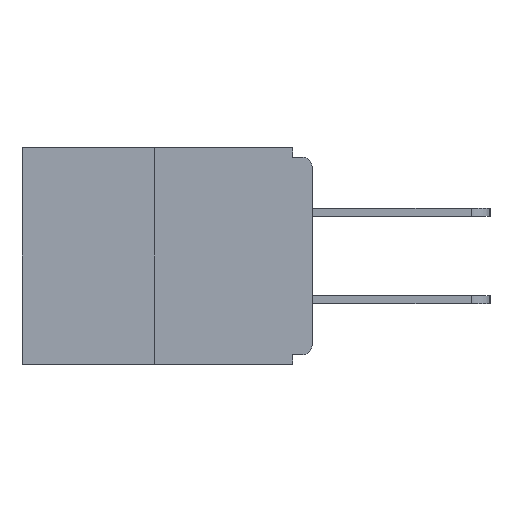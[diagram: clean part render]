
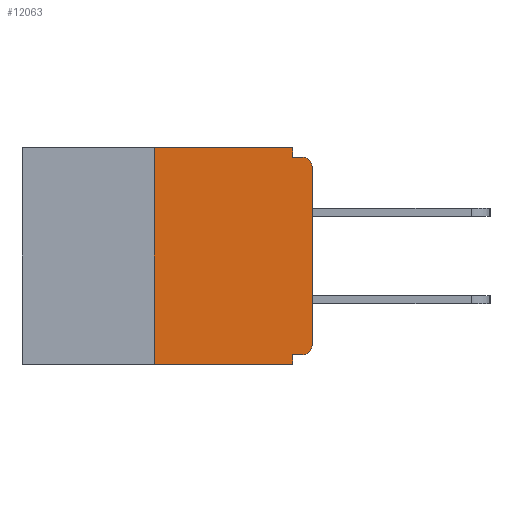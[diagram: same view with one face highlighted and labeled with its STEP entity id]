
A CAD part, left-side view. The second image highlights one B-rep face of the part: STEP entity #12063.
In plain terms, the highlighted planar face has unit normal (-1, 0, 0).
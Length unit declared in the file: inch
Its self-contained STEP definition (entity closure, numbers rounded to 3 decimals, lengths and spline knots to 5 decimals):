
#391 = CARTESIAN_POINT ( 'NONE',  ( 0., 0., -0.313 ) ) ;
#1004 = CARTESIAN_POINT ( 'NONE',  ( 0., 0.25, -0.343 ) ) ;
#1008 = ORIENTED_EDGE ( 'NONE', *, *, #11610, .T. ) ;
#1175 = EDGE_CURVE ( 'NONE', #9377, #4751, #9925, .T. ) ;
#1349 = DIRECTION ( 'NONE',  ( 0., -1., 0. ) ) ;
#1605 = PLANE ( 'NONE',  #22102 ) ;
#1677 = CARTESIAN_POINT ( 'NONE',  ( 0., 0.25, 0. ) ) ;
#2037 = DIRECTION ( 'NONE',  ( 0., -1., 0. ) ) ;
#2248 = VERTEX_POINT ( 'NONE', #4622 ) ;
#2305 = CARTESIAN_POINT ( 'NONE',  ( 0., 0., -0.328 ) ) ;
#2368 = EDGE_CURVE ( 'NONE', #2248, #4751, #23819, .T. ) ;
#2661 = LINE ( 'NONE', #3225, #23121 ) ;
#3225 = CARTESIAN_POINT ( 'NONE',  ( 0., 0., 0. ) ) ;
#3292 = EDGE_CURVE ( 'NONE', #3612, #2248, #24144, .T. ) ;
#3564 = CARTESIAN_POINT ( 'NONE',  ( 0., 0.46, 0. ) ) ;
#3612 = VERTEX_POINT ( 'NONE', #6623 ) ;
#3667 = DIRECTION ( 'NONE',  ( -1., 0., 0. ) ) ;
#3917 = CIRCLE ( 'NONE', #20356, 0.015 ) ;
#4182 = FACE_OUTER_BOUND ( 'NONE', #16368, .T. ) ;
#4429 = VECTOR ( 'NONE', #14048, 39.37008 ) ;
#4442 = EDGE_CURVE ( 'NONE', #17033, #9377, #2661, .T. ) ;
#4622 = CARTESIAN_POINT ( 'NONE',  ( 0., 0.031, -0.015 ) ) ;
#4633 = DIRECTION ( 'NONE',  ( 0., -1., 0. ) ) ;
#4751 = VERTEX_POINT ( 'NONE', #19580 ) ;
#4884 = VECTOR ( 'NONE', #13050, 39.37008 ) ;
#5067 = CARTESIAN_POINT ( 'NONE',  ( 0., 0., -0.015 ) ) ;
#5265 = VECTOR ( 'NONE', #12863, 39.37008 ) ;
#5357 = VERTEX_POINT ( 'NONE', #9931 ) ;
#5577 = DIRECTION ( 'NONE',  ( 0., 0., -1. ) ) ;
#5668 = DIRECTION ( 'NONE',  ( 0., 0., -1. ) ) ;
#6623 = CARTESIAN_POINT ( 'NONE',  ( 0., 0.031, 0. ) ) ;
#6830 = EDGE_CURVE ( 'NONE', #8139, #20433, #11661, .T. ) ;
#7882 = EDGE_CURVE ( 'NONE', #5357, #12253, #8182, .T. ) ;
#8139 = VERTEX_POINT ( 'NONE', #1004 ) ;
#8182 = LINE ( 'NONE', #2305, #4429 ) ;
#9209 = CARTESIAN_POINT ( 'NONE',  ( 0., 0.015, -0.313 ) ) ;
#9355 = EDGE_CURVE ( 'NONE', #19611, #3612, #9945, .T. ) ;
#9377 = VERTEX_POINT ( 'NONE', #18538 ) ;
#9925 = CIRCLE ( 'NONE', #15510, 0.015 ) ;
#9931 = CARTESIAN_POINT ( 'NONE',  ( 0., 0.015, -0.328 ) ) ;
#9945 = LINE ( 'NONE', #24041, #19563 ) ;
#10137 = CARTESIAN_POINT ( 'NONE',  ( 0., 0.031, -0.343 ) ) ;
#10160 = EDGE_CURVE ( 'NONE', #8139, #19611, #24498, .T. ) ;
#10308 = LINE ( 'NONE', #10137, #18350 ) ;
#11610 = EDGE_CURVE ( 'NONE', #5357, #17033, #3917, .T. ) ;
#11657 = ORIENTED_EDGE ( 'NONE', *, *, #4442, .T. ) ;
#11661 = LINE ( 'NONE', #12591, #23129 ) ;
#11884 = ORIENTED_EDGE ( 'NONE', *, *, #10160, .F. ) ;
#12063 = ADVANCED_FACE ( 'NONE', ( #4182 ), #1605, .F. ) ;
#12253 = VERTEX_POINT ( 'NONE', #17730 ) ;
#12591 = CARTESIAN_POINT ( 'NONE',  ( 0., 0.46, -0.343 ) ) ;
#12810 = DIRECTION ( 'NONE',  ( 0., 0., 1. ) ) ;
#12863 = DIRECTION ( 'NONE',  ( 0., 0., 1. ) ) ;
#12953 = CARTESIAN_POINT ( 'NONE',  ( 0., 0.25, 0. ) ) ;
#13050 = DIRECTION ( 'NONE',  ( 0., 0., -1. ) ) ;
#13187 = DIRECTION ( 'NONE',  ( -1., 0., 0. ) ) ;
#14048 = DIRECTION ( 'NONE',  ( 0., 1., 0. ) ) ;
#15510 = AXIS2_PLACEMENT_3D ( 'NONE', #23530, #3667, #5668 ) ;
#16341 = DIRECTION ( 'NONE',  ( 0., 0., -1. ) ) ;
#16368 = EDGE_LOOP ( 'NONE', ( #20426, #11884, #22947, #25369, #23809, #1008, #11657, #19366, #23093, #24307 ) ) ;
#17033 = VERTEX_POINT ( 'NONE', #391 ) ;
#17323 = CARTESIAN_POINT ( 'NONE',  ( 0., 0.031, -0.343 ) ) ;
#17730 = CARTESIAN_POINT ( 'NONE',  ( 0., 0.031, -0.328 ) ) ;
#18350 = VECTOR ( 'NONE', #16341, 39.37008 ) ;
#18538 = CARTESIAN_POINT ( 'NONE',  ( 0., 0., -0.03 ) ) ;
#19248 = DIRECTION ( 'NONE',  ( 1., 0., 0. ) ) ;
#19366 = ORIENTED_EDGE ( 'NONE', *, *, #1175, .T. ) ;
#19563 = VECTOR ( 'NONE', #2037, 39.37008 ) ;
#19580 = CARTESIAN_POINT ( 'NONE',  ( 0., 0.015, -0.015 ) ) ;
#19611 = VERTEX_POINT ( 'NONE', #1677 ) ;
#20356 = AXIS2_PLACEMENT_3D ( 'NONE', #9209, #13187, #23086 ) ;
#20426 = ORIENTED_EDGE ( 'NONE', *, *, #9355, .F. ) ;
#20433 = VERTEX_POINT ( 'NONE', #17323 ) ;
#22102 = AXIS2_PLACEMENT_3D ( 'NONE', #3564, #19248, #5577 ) ;
#22947 = ORIENTED_EDGE ( 'NONE', *, *, #6830, .T. ) ;
#23086 = DIRECTION ( 'NONE',  ( 0., 0., -1. ) ) ;
#23093 = ORIENTED_EDGE ( 'NONE', *, *, #2368, .F. ) ;
#23121 = VECTOR ( 'NONE', #12810, 39.37008 ) ;
#23129 = VECTOR ( 'NONE', #4633, 39.37008 ) ;
#23195 = EDGE_CURVE ( 'NONE', #12253, #20433, #10308, .T. ) ;
#23530 = CARTESIAN_POINT ( 'NONE',  ( 0., 0.015, -0.03 ) ) ;
#23809 = ORIENTED_EDGE ( 'NONE', *, *, #7882, .F. ) ;
#23819 = LINE ( 'NONE', #5067, #24455 ) ;
#24041 = CARTESIAN_POINT ( 'NONE',  ( 0., 0.46, 0. ) ) ;
#24144 = LINE ( 'NONE', #25082, #4884 ) ;
#24307 = ORIENTED_EDGE ( 'NONE', *, *, #3292, .F. ) ;
#24455 = VECTOR ( 'NONE', #1349, 39.37008 ) ;
#24498 = LINE ( 'NONE', #12953, #5265 ) ;
#25082 = CARTESIAN_POINT ( 'NONE',  ( 0., 0.031, 0. ) ) ;
#25369 = ORIENTED_EDGE ( 'NONE', *, *, #23195, .F. ) ;
